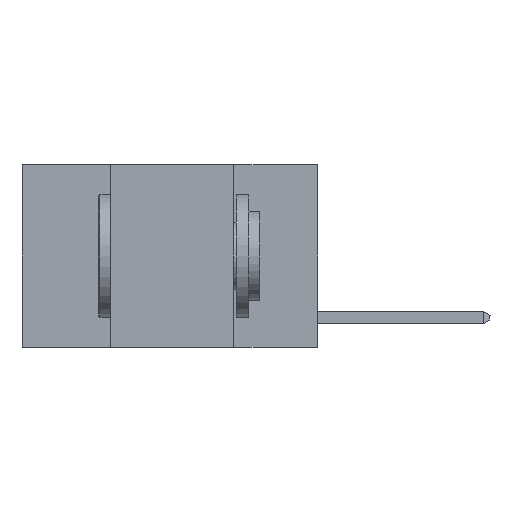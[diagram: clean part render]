
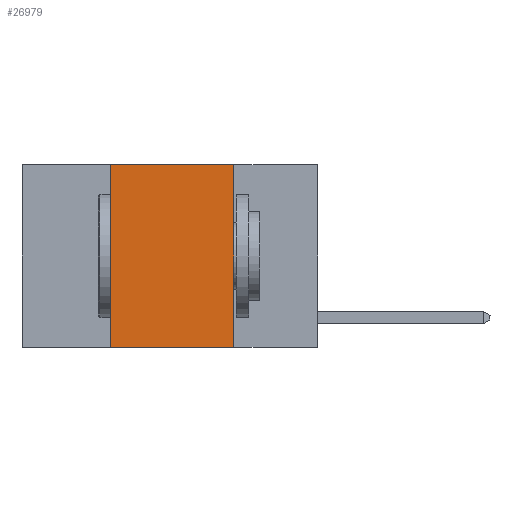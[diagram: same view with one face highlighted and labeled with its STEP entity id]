
A CAD part, left-side view. The second image highlights one B-rep face of the part: STEP entity #26979.
In plain terms, the highlighted planar face has unit normal (-1, 0, 0).
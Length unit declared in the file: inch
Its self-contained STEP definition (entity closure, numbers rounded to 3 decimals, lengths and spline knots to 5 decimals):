
#339 = EDGE_CURVE ( 'NONE', #3366, #12995, #21972, .T. ) ;
#433 = DIRECTION ( 'NONE',  ( 1., 0., 0. ) ) ;
#571 = CARTESIAN_POINT ( 'NONE',  ( 0., 0.6, 0. ) ) ;
#1618 = ORIENTED_EDGE ( 'NONE', *, *, #20187, .F. ) ;
#2818 = LINE ( 'NONE', #23587, #12943 ) ;
#3366 = VERTEX_POINT ( 'NONE', #23201 ) ;
#4060 = ORIENTED_EDGE ( 'NONE', *, *, #25562, .T. ) ;
#4088 = ORIENTED_EDGE ( 'NONE', *, *, #339, .F. ) ;
#4199 = DIRECTION ( 'NONE',  ( 0., -1., 0. ) ) ;
#4636 = EDGE_LOOP ( 'NONE', ( #1618, #17208, #4088, #4060 ) ) ;
#8131 = EDGE_CURVE ( 'NONE', #12995, #13171, #2818, .T. ) ;
#8285 = CARTESIAN_POINT ( 'NONE',  ( 0., 0.17, -0.37 ) ) ;
#9102 = VERTEX_POINT ( 'NONE', #8285 ) ;
#9318 = LINE ( 'NONE', #23001, #26331 ) ;
#9433 = CARTESIAN_POINT ( 'NONE',  ( 0., 0.42, 0. ) ) ;
#9887 = DIRECTION ( 'NONE',  ( 0., -1., 0. ) ) ;
#11767 = VECTOR ( 'NONE', #19714, 39.37008 ) ;
#12018 = FACE_OUTER_BOUND ( 'NONE', #4636, .T. ) ;
#12300 = PLANE ( 'NONE',  #23438 ) ;
#12943 = VECTOR ( 'NONE', #9887, 39.37008 ) ;
#12995 = VERTEX_POINT ( 'NONE', #9433 ) ;
#13171 = VERTEX_POINT ( 'NONE', #21614 ) ;
#14682 = DIRECTION ( 'NONE',  ( 0., 0., -1. ) ) ;
#16664 = DIRECTION ( 'NONE',  ( 0., 0., -1. ) ) ;
#17208 = ORIENTED_EDGE ( 'NONE', *, *, #8131, .F. ) ;
#19714 = DIRECTION ( 'NONE',  ( 0., 0., 1. ) ) ;
#20187 = EDGE_CURVE ( 'NONE', #13171, #9102, #25594, .T. ) ;
#20888 = VECTOR ( 'NONE', #14682, 39.37008 ) ;
#21614 = CARTESIAN_POINT ( 'NONE',  ( 0., 0.17, 0. ) ) ;
#21972 = LINE ( 'NONE', #26337, #11767 ) ;
#23001 = CARTESIAN_POINT ( 'NONE',  ( 0., 0.6, -0.37 ) ) ;
#23201 = CARTESIAN_POINT ( 'NONE',  ( 0., 0.42, -0.37 ) ) ;
#23438 = AXIS2_PLACEMENT_3D ( 'NONE', #571, #433, #16664 ) ;
#23587 = CARTESIAN_POINT ( 'NONE',  ( 0., 0.6, 0. ) ) ;
#23740 = CARTESIAN_POINT ( 'NONE',  ( 0., 0.17, 0. ) ) ;
#25562 = EDGE_CURVE ( 'NONE', #3366, #9102, #9318, .T. ) ;
#25594 = LINE ( 'NONE', #23740, #20888 ) ;
#26331 = VECTOR ( 'NONE', #4199, 39.37008 ) ;
#26337 = CARTESIAN_POINT ( 'NONE',  ( 0., 0.42, 0. ) ) ;
#26979 = ADVANCED_FACE ( 'NONE', ( #12018 ), #12300, .F. ) ;
